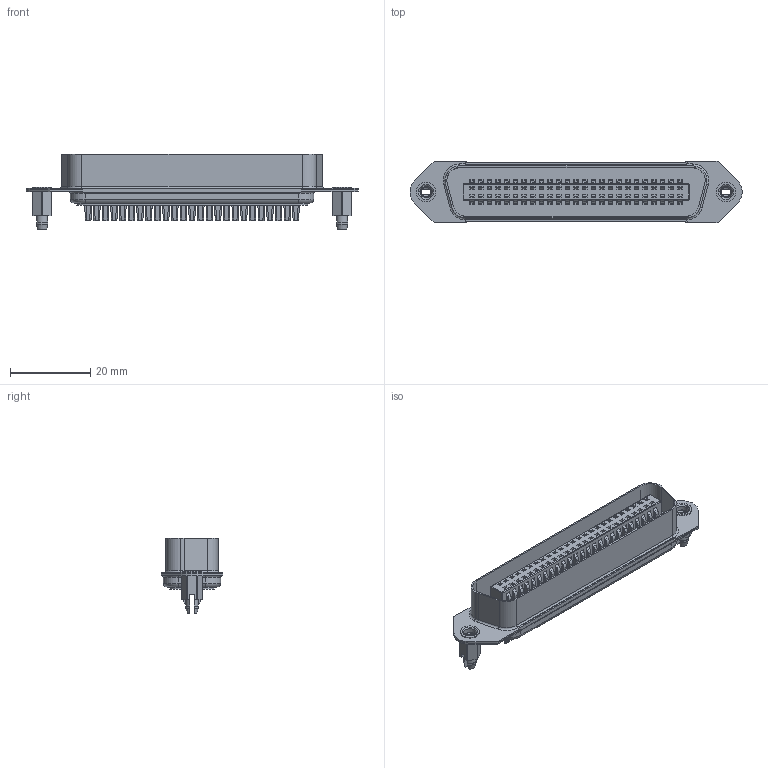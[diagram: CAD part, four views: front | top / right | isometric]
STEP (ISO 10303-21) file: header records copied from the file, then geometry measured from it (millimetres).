
FILE_DESCRIPTION (( 'STEP AP203' ), '1' );
FILE_NAME ('B57-150-622-502.STEP', '2020-06-24T12:43:13', ( '' ), ( '' ), 'SwSTEP 2.0', 'SolidWorks 2020', '' );
FILE_SCHEMA (( 'CONFIG_CONTROL_DESIGN' ));
Length unit declared in the file: millimetre
Products named in the file (6): B57 Housing Insert MALE_50 Position UP; B57 Front Shell MALE_50 Position UP; B57 Back Shell_50 Position; B57-150-622-502; B57 Contacts MALE_50 Position SOLDER; B57 Rivet_STR THREAD BOARDLOCK 
Assembly tree (6 placements, depth 2):
  B57-150-622-502
    B57 Back Shell_50 Position
    B57 Rivet_STR THREAD BOARDLOCK   x2
    B57 Housing Insert MALE_50 Position UP
    B57 Front Shell MALE_50 Position UP
    B57 Contacts MALE_50 Position SOLDER
Bounding box: 82.83 x 15.3 x 18.8 mm (x, y, z)
Volume: 6069 mm3; surface area: 15070.2 mm2
Topology: 55 solids, 55 shells, 5343 faces, 15211 edges, 9680 vertices
Faces by surface type: plane 3805, cylinder 1280, sphere 204, torus 30, cone 14, bspline 10
Entity records: 171550 total; most frequent: CARTESIAN_POINT 34844, ORIENTED_EDGE 29640, DIRECTION 26795, EDGE_CURVE 14820, VECTOR 11835, LINE 11835, VERTEX_POINT 9556, AXIS2_PLACEMENT_3D 7480
